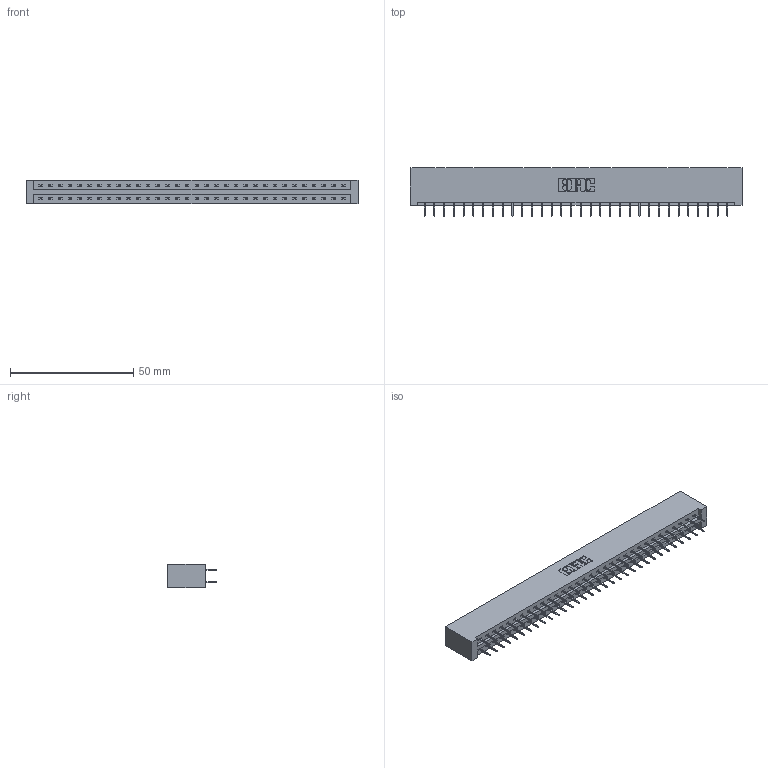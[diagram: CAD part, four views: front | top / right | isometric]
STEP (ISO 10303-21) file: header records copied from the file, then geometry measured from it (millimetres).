
FILE_DESCRIPTION (( 'STEP AP203' ), '1' );
FILE_NAME ('387-064-524-201.STEP', '2018-09-21T07:10:14', ( '' ), ( '' ), 'SwSTEP 2.0', 'SolidWorks 2016', '' );
FILE_SCHEMA (( 'CONFIG_CONTROL_DESIGN' ));
Length unit declared in the file: inch
Products named in the file (3): 345-292-001_345-293-124; 387-064-524-201; 337 Part_No Mounting Lugs
Assembly tree (65 placements, depth 2):
  387-064-524-201
    337 Part_No Mounting Lugs
    345-292-001_345-293-124  x64
Bounding box: 134.67 x 19.69 x 9.4 mm (x, y, z)
Volume: 14723.5 mm3; surface area: 16303.9 mm2
Topology: 65 solids, 65 shells, 3818 faces, 10847 edges, 6974 vertices
Faces by surface type: plane 2882, cylinder 936
Entity records: 25901 total; most frequent: CARTESIAN_POINT 4370, ORIENTED_EDGE 4306, DIRECTION 3729, EDGE_CURVE 2153, VECTOR 2037, LINE 2037, VERTEX_POINT 1430, AXIS2_PLACEMENT_3D 846
